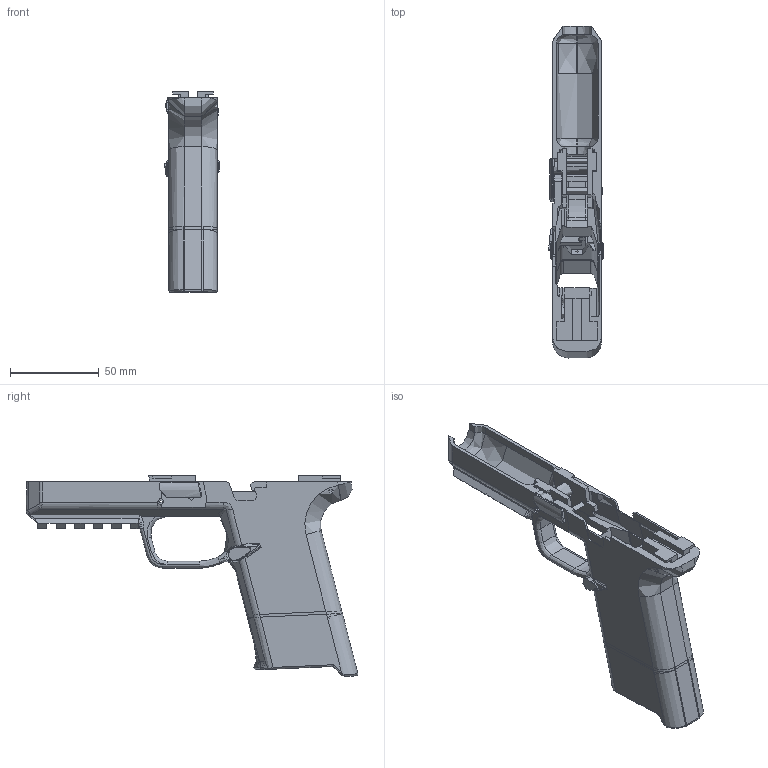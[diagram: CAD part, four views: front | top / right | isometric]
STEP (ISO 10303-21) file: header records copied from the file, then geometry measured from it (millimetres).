
FILE_DESCRIPTION(/* description */ (''),/* implementation_level */ '2;1');
FILE_NAME(/* name */ 'M&P 9 Assembly + Picatinny - Full Size Slide.step',/* time_stamp */ '2022-01-06T22:54:17-05:00',/* author */ (''),/* organization */ (''),/* preprocessor_version */ 'ST-DEVELOPER v18.1',/* originating_system */ 'Autodesk Translation Framework v10.10.0.1391',/* authorisation */ '');
FILE_SCHEMA (('AUTOMOTIVE_DESIGN { 1 0 10303 214 3 1 1 }'));
Length unit declared in the file: millimetre
Products named in the file (14): M&P 9 Standard Length Slide - Picatinny; M&P 9 Reference v114; Rear Fire Control Group Pin; Front Locking Block Group Pin; Trigger Pin; Locking Block; Disassembly Lug; Rear Fire Control Group; Frame; Trigger Guard and Magwell; Fitment Section; M1.0 Full-size Nose; Full-Size Magwell Body; Magazine Release Button
Assembly tree (13 placements, depth 5):
  M&P 9 Standard Length Slide - Picatinny
    M&P 9 Reference v114
      Rear Fire Control Group Pin
      Front Locking Block Group Pin
      Trigger Pin
      Locking Block
      Disassembly Lug
      Rear Fire Control Group
      Frame
        Trigger Guard and Magwell
        Fitment Section
          M1.0 Full-size Nose
        Full-Size Magwell Body
      Magazine Release Button
Bounding box: 30.95 x 186.75 x 113.13 mm (x, y, z)
Volume: 108681.9 mm3; surface area: 59061.8 mm2
Topology: 11 solids, 11 shells, 739 faces, 2002 edges, 1270 vertices
Faces by surface type: plane 380, cylinder 208, bspline 124, torus 21, sphere 4, cone 2
Full cylindrical faces by diameter (mm): 1.35 x2, 1.5 x3, 3.15 x2, 3.18 x3, 3.2 x2, 3.361 x2, 3.5 x1, 3.55 x4, 4.7 x1, 5.1 x1, 6.3 x1, 7.7 x1, 8.8 x1, 9 x2
Entity records: 27575 total; most frequent: CARTESIAN_POINT 8981, ORIENTED_EDGE 3982, DIRECTION 3581, EDGE_CURVE 1991, VERTEX_POINT 1270, LINE 1195, VECTOR 1195, AXIS2_PLACEMENT_3D 1193
